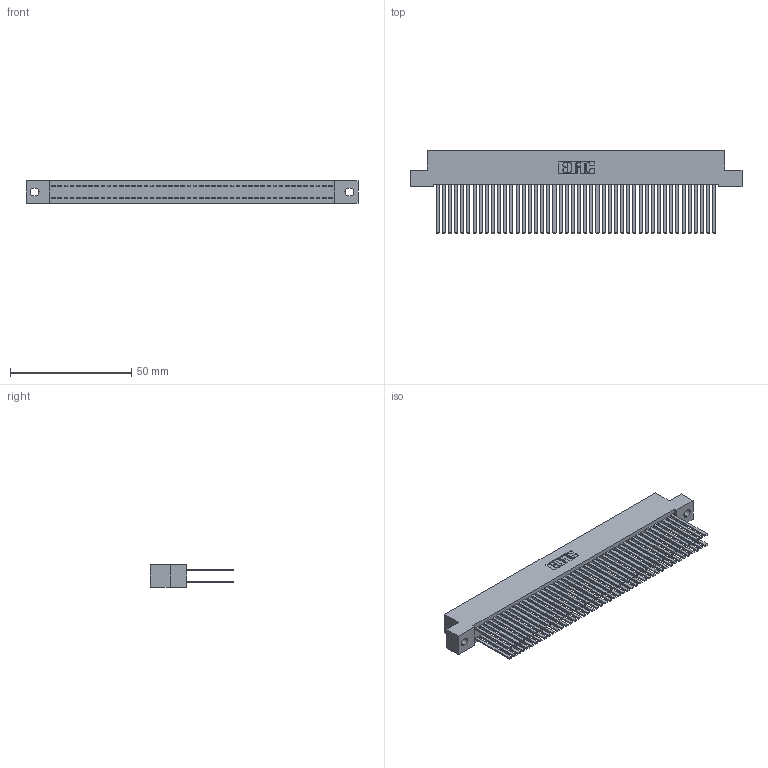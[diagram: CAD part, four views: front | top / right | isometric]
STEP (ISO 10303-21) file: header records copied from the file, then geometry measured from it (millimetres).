
FILE_DESCRIPTION (( 'STEP AP203' ), '1' );
FILE_NAME ('392-092-544-202.STEP', '2019-10-09T18:58:17', ( '' ), ( '' ), 'SwSTEP 2.0', 'SolidWorks 2016', '' );
FILE_SCHEMA (( 'CONFIG_CONTROL_DESIGN' ));
Length unit declared in the file: inch
Products named in the file (3): 342 Part_.128 Slot; 345-292-001_345-293-144; 392-092-544-202
Assembly tree (93 placements, depth 2):
  392-092-544-202
    342 Part_.128 Slot
    345-292-001_345-293-144  x92
Bounding box: 137.16 x 34.3 x 9.4 mm (x, y, z)
Volume: 13580.3 mm3; surface area: 25534.9 mm2
Topology: 93 solids, 93 shells, 4346 faces, 12915 edges, 8486 vertices
Faces by surface type: plane 3014, cylinder 1332
Entity records: 28895 total; most frequent: CARTESIAN_POINT 4782, ORIENTED_EDGE 4718, DIRECTION 4075, EDGE_CURVE 2359, VECTOR 2235, LINE 2235, VERTEX_POINT 1570, AXIS2_PLACEMENT_3D 920
